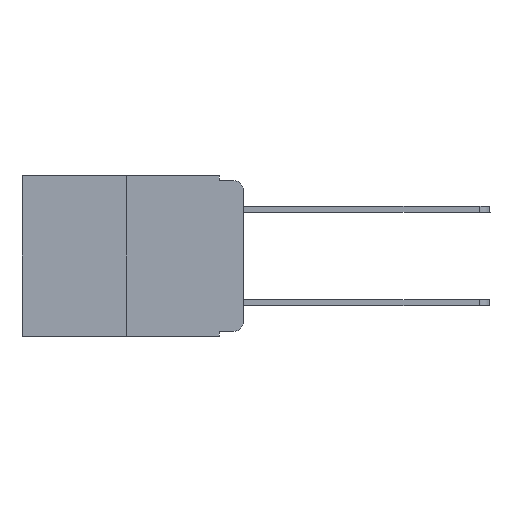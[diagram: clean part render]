
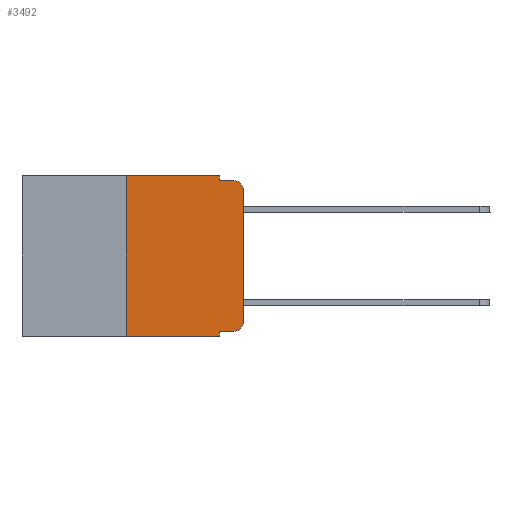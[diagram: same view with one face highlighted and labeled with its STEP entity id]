
A CAD part, left-side view. The second image highlights one B-rep face of the part: STEP entity #3492.
In plain terms, the highlighted planar face has unit normal (-1, 0, 0).
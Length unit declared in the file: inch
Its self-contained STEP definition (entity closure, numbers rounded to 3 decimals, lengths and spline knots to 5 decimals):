
#907 = VERTEX_POINT ( 'NONE', #1320 ) ;
#949 = ORIENTED_EDGE ( 'NONE', *, *, #14811, .F. ) ;
#1320 = CARTESIAN_POINT ( 'NONE',  ( 0., 0.051, -0.01 ) ) ;
#2176 = CARTESIAN_POINT ( 'NONE',  ( 0., 0.25, -0.343 ) ) ;
#2186 = DIRECTION ( 'NONE',  ( 1., 0., 0. ) ) ;
#2607 = CARTESIAN_POINT ( 'NONE',  ( 0., 0.473, -0.343 ) ) ;
#2868 = DIRECTION ( 'NONE',  ( 0., -1., 0. ) ) ;
#2870 = CARTESIAN_POINT ( 'NONE',  ( 0., 0., -0.03 ) ) ;
#3228 = AXIS2_PLACEMENT_3D ( 'NONE', #17018, #18538, #12297 ) ;
#3286 = VERTEX_POINT ( 'NONE', #2870 ) ;
#3492 = ADVANCED_FACE ( 'NONE', ( #8813 ), #9644, .F. ) ;
#3541 = EDGE_CURVE ( 'NONE', #16393, #9669, #3980, .T. ) ;
#3629 = ORIENTED_EDGE ( 'NONE', *, *, #18349, .T. ) ;
#3920 = EDGE_CURVE ( 'NONE', #13526, #8730, #19519, .T. ) ;
#3980 = LINE ( 'NONE', #19033, #12763 ) ;
#4150 = DIRECTION ( 'NONE',  ( 0., -1., 0. ) ) ;
#4421 = VECTOR ( 'NONE', #4150, 39.37008 ) ;
#4430 = CARTESIAN_POINT ( 'NONE',  ( 0., 0.051, 0. ) ) ;
#4623 = LINE ( 'NONE', #4430, #11911 ) ;
#5048 = LINE ( 'NONE', #9202, #15962 ) ;
#5188 = VECTOR ( 'NONE', #2868, 39.37008 ) ;
#5219 = CARTESIAN_POINT ( 'NONE',  ( 0., 0.473, 0. ) ) ;
#5417 = DIRECTION ( 'NONE',  ( -1., 0., 0. ) ) ;
#5543 = VERTEX_POINT ( 'NONE', #15461 ) ;
#5771 = AXIS2_PLACEMENT_3D ( 'NONE', #5219, #2186, #16129 ) ;
#6003 = ORIENTED_EDGE ( 'NONE', *, *, #16453, .T. ) ;
#7549 = DIRECTION ( 'NONE',  ( 0., 0., -1. ) ) ;
#8556 = DIRECTION ( 'NONE',  ( 0., 0., -1. ) ) ;
#8730 = VERTEX_POINT ( 'NONE', #15455 ) ;
#8802 = VECTOR ( 'NONE', #15054, 39.37008 ) ;
#8813 = FACE_OUTER_BOUND ( 'NONE', #9133, .T. ) ;
#9133 = EDGE_LOOP ( 'NONE', ( #18595, #3629, #14220, #10216, #15938, #949, #6003, #14783, #16841, #14901 ) ) ;
#9159 = CARTESIAN_POINT ( 'NONE',  ( 0., 0.02, -0.333 ) ) ;
#9202 = CARTESIAN_POINT ( 'NONE',  ( 0., 0., 0. ) ) ;
#9225 = VERTEX_POINT ( 'NONE', #2176 ) ;
#9281 = VECTOR ( 'NONE', #12681, 39.37008 ) ;
#9531 = LINE ( 'NONE', #2607, #4421 ) ;
#9644 = PLANE ( 'NONE',  #5771 ) ;
#9669 = VERTEX_POINT ( 'NONE', #11202 ) ;
#9705 = DIRECTION ( 'NONE',  ( 0., 0., -1. ) ) ;
#9787 = LINE ( 'NONE', #15704, #9281 ) ;
#10216 = ORIENTED_EDGE ( 'NONE', *, *, #11294, .F. ) ;
#10761 = VECTOR ( 'NONE', #16509, 39.37008 ) ;
#11113 = VERTEX_POINT ( 'NONE', #16928 ) ;
#11202 = CARTESIAN_POINT ( 'NONE',  ( 0., 0.051, -0.343 ) ) ;
#11294 = EDGE_CURVE ( 'NONE', #15782, #907, #4623, .T. ) ;
#11911 = VECTOR ( 'NONE', #7549, 39.37008 ) ;
#12223 = DIRECTION ( 'NONE',  ( 0., 0., 1. ) ) ;
#12297 = DIRECTION ( 'NONE',  ( 0., 0., -1. ) ) ;
#12487 = LINE ( 'NONE', #16761, #8802 ) ;
#12681 = DIRECTION ( 'NONE',  ( 0., -1., 0. ) ) ;
#12763 = VECTOR ( 'NONE', #9705, 39.37008 ) ;
#13526 = VERTEX_POINT ( 'NONE', #9159 ) ;
#13912 = EDGE_CURVE ( 'NONE', #11113, #15782, #19801, .T. ) ;
#14100 = EDGE_CURVE ( 'NONE', #907, #5543, #15600, .T. ) ;
#14220 = ORIENTED_EDGE ( 'NONE', *, *, #14100, .F. ) ;
#14783 = ORIENTED_EDGE ( 'NONE', *, *, #3541, .F. ) ;
#14811 = EDGE_CURVE ( 'NONE', #9225, #11113, #12487, .T. ) ;
#14901 = ORIENTED_EDGE ( 'NONE', *, *, #3920, .T. ) ;
#15054 = DIRECTION ( 'NONE',  ( 0., 0., 1. ) ) ;
#15455 = CARTESIAN_POINT ( 'NONE',  ( 0., 0., -0.313 ) ) ;
#15461 = CARTESIAN_POINT ( 'NONE',  ( 0., 0.02, -0.01 ) ) ;
#15600 = LINE ( 'NONE', #19618, #10761 ) ;
#15704 = CARTESIAN_POINT ( 'NONE',  ( 0., 0.051, -0.333 ) ) ;
#15782 = VERTEX_POINT ( 'NONE', #15963 ) ;
#15788 = AXIS2_PLACEMENT_3D ( 'NONE', #17858, #5417, #8556 ) ;
#15938 = ORIENTED_EDGE ( 'NONE', *, *, #13912, .F. ) ;
#15962 = VECTOR ( 'NONE', #12223, 39.37008 ) ;
#15963 = CARTESIAN_POINT ( 'NONE',  ( 0., 0.051, 0. ) ) ;
#16129 = DIRECTION ( 'NONE',  ( 0., 0., -1. ) ) ;
#16393 = VERTEX_POINT ( 'NONE', #19932 ) ;
#16453 = EDGE_CURVE ( 'NONE', #9225, #9669, #9531, .T. ) ;
#16509 = DIRECTION ( 'NONE',  ( 0., -1., 0. ) ) ;
#16761 = CARTESIAN_POINT ( 'NONE',  ( 0., 0.25, 0. ) ) ;
#16841 = ORIENTED_EDGE ( 'NONE', *, *, #19293, .T. ) ;
#16928 = CARTESIAN_POINT ( 'NONE',  ( 0., 0.25, 0. ) ) ;
#17018 = CARTESIAN_POINT ( 'NONE',  ( 0., 0.02, -0.313 ) ) ;
#17858 = CARTESIAN_POINT ( 'NONE',  ( 0., 0.02, -0.03 ) ) ;
#18192 = CIRCLE ( 'NONE', #15788, 0.02 ) ;
#18349 = EDGE_CURVE ( 'NONE', #3286, #5543, #18192, .T. ) ;
#18538 = DIRECTION ( 'NONE',  ( -1., 0., 0. ) ) ;
#18595 = ORIENTED_EDGE ( 'NONE', *, *, #19548, .T. ) ;
#19033 = CARTESIAN_POINT ( 'NONE',  ( 0., 0.051, 0. ) ) ;
#19293 = EDGE_CURVE ( 'NONE', #16393, #13526, #9787, .T. ) ;
#19519 = CIRCLE ( 'NONE', #3228, 0.02 ) ;
#19548 = EDGE_CURVE ( 'NONE', #8730, #3286, #5048, .T. ) ;
#19618 = CARTESIAN_POINT ( 'NONE',  ( 0., 0.051, -0.01 ) ) ;
#19801 = LINE ( 'NONE', #19997, #5188 ) ;
#19932 = CARTESIAN_POINT ( 'NONE',  ( 0., 0.051, -0.333 ) ) ;
#19997 = CARTESIAN_POINT ( 'NONE',  ( 0., 0.473, 0. ) ) ;
